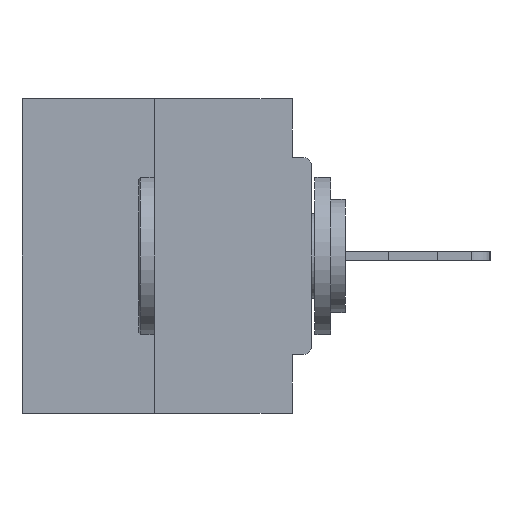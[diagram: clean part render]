
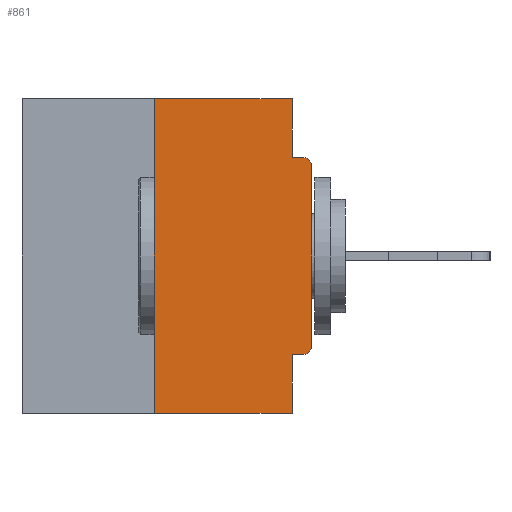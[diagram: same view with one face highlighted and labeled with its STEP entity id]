
A CAD part, left-side view. The second image highlights one B-rep face of the part: STEP entity #861.
In plain terms, the highlighted planar face has unit normal (-1, 0, 0).
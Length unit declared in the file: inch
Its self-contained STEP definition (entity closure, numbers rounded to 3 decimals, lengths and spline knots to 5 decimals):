
#429 = VERTEX_POINT ( 'NONE', #19934 ) ;
#861 = ADVANCED_FACE ( 'NONE', ( #7298 ), #9943, .F. ) ;
#922 = CARTESIAN_POINT ( 'NONE',  ( 0., 0.46, 0. ) ) ;
#953 = LINE ( 'NONE', #10120, #7994 ) ;
#1533 = DIRECTION ( 'NONE',  ( -1., 0., 0. ) ) ;
#2012 = VERTEX_POINT ( 'NONE', #7762 ) ;
#2279 = VERTEX_POINT ( 'NONE', #18960 ) ;
#2913 = DIRECTION ( 'NONE',  ( 0., 0., 1. ) ) ;
#3044 = VERTEX_POINT ( 'NONE', #5951 ) ;
#3590 = LINE ( 'NONE', #22422, #23244 ) ;
#3699 = CARTESIAN_POINT ( 'NONE',  ( 0., 0., -0.1085 ) ) ;
#4119 = EDGE_CURVE ( 'NONE', #4155, #16499, #11860, .T. ) ;
#4155 = VERTEX_POINT ( 'NONE', #9522 ) ;
#4285 = ORIENTED_EDGE ( 'NONE', *, *, #11228, .T. ) ;
#5045 = EDGE_LOOP ( 'NONE', ( #5771, #16058, #4285, #12949, #11270, #27238, #19919, #18585, #28527, #9793 ) ) ;
#5436 = LINE ( 'NONE', #27053, #20895 ) ;
#5771 = ORIENTED_EDGE ( 'NONE', *, *, #6551, .F. ) ;
#5951 = CARTESIAN_POINT ( 'NONE',  ( 0., 0.031, -0.4065 ) ) ;
#6551 = EDGE_CURVE ( 'NONE', #2012, #7113, #3590, .T. ) ;
#6617 = CARTESIAN_POINT ( 'NONE',  ( 0., 0.031, -0.0935 ) ) ;
#6985 = AXIS2_PLACEMENT_3D ( 'NONE', #7805, #1533, #22107 ) ;
#7113 = VERTEX_POINT ( 'NONE', #11018 ) ;
#7218 = VECTOR ( 'NONE', #21047, 39.37008 ) ;
#7298 = FACE_OUTER_BOUND ( 'NONE', #5045, .T. ) ;
#7762 = CARTESIAN_POINT ( 'NONE',  ( 0., 0.25, 0. ) ) ;
#7805 = CARTESIAN_POINT ( 'NONE',  ( 0., 0.015, -0.1085 ) ) ;
#7994 = VECTOR ( 'NONE', #25486, 39.37008 ) ;
#8562 = DIRECTION ( 'NONE',  ( 0., -1., 0. ) ) ;
#9522 = CARTESIAN_POINT ( 'NONE',  ( 0., 0., -0.3915 ) ) ;
#9664 = CARTESIAN_POINT ( 'NONE',  ( 0., 0., 0. ) ) ;
#9793 = ORIENTED_EDGE ( 'NONE', *, *, #26928, .F. ) ;
#9943 = PLANE ( 'NONE',  #16015 ) ;
#10120 = CARTESIAN_POINT ( 'NONE',  ( 0., 0.46, -0.5 ) ) ;
#10135 = LINE ( 'NONE', #22425, #25837 ) ;
#11018 = CARTESIAN_POINT ( 'NONE',  ( 0., 0.031, 0. ) ) ;
#11034 = VECTOR ( 'NONE', #20448, 39.37008 ) ;
#11209 = CARTESIAN_POINT ( 'NONE',  ( 0., 0.015, -0.3915 ) ) ;
#11228 = EDGE_CURVE ( 'NONE', #17692, #16939, #953, .T. ) ;
#11270 = ORIENTED_EDGE ( 'NONE', *, *, #23505, .F. ) ;
#11860 = LINE ( 'NONE', #9664, #7218 ) ;
#12949 = ORIENTED_EDGE ( 'NONE', *, *, #21204, .F. ) ;
#14270 = CARTESIAN_POINT ( 'NONE',  ( 0., 0.25, 0. ) ) ;
#15337 = CARTESIAN_POINT ( 'NONE',  ( 0., 0.031, -0.5 ) ) ;
#16015 = AXIS2_PLACEMENT_3D ( 'NONE', #922, #26295, #19442 ) ;
#16035 = DIRECTION ( 'NONE',  ( 0., 0., -1. ) ) ;
#16058 = ORIENTED_EDGE ( 'NONE', *, *, #16781, .F. ) ;
#16499 = VERTEX_POINT ( 'NONE', #3699 ) ;
#16549 = EDGE_CURVE ( 'NONE', #16499, #429, #27867, .T. ) ;
#16781 = EDGE_CURVE ( 'NONE', #17692, #2012, #23922, .T. ) ;
#16939 = VERTEX_POINT ( 'NONE', #15337 ) ;
#16960 = DIRECTION ( 'NONE',  ( 0., 0., -1. ) ) ;
#17440 = VECTOR ( 'NONE', #2913, 39.37008 ) ;
#17692 = VERTEX_POINT ( 'NONE', #30551 ) ;
#18066 = EDGE_CURVE ( 'NONE', #2279, #4155, #28645, .T. ) ;
#18364 = LINE ( 'NONE', #23180, #30116 ) ;
#18585 = ORIENTED_EDGE ( 'NONE', *, *, #16549, .T. ) ;
#18960 = CARTESIAN_POINT ( 'NONE',  ( 0., 0.015, -0.4065 ) ) ;
#19193 = AXIS2_PLACEMENT_3D ( 'NONE', #11209, #20717, #16035 ) ;
#19442 = DIRECTION ( 'NONE',  ( 0., 0., -1. ) ) ;
#19919 = ORIENTED_EDGE ( 'NONE', *, *, #4119, .T. ) ;
#19934 = CARTESIAN_POINT ( 'NONE',  ( 0., 0.015, -0.0935 ) ) ;
#20448 = DIRECTION ( 'NONE',  ( 0., 1., 0. ) ) ;
#20717 = DIRECTION ( 'NONE',  ( -1., 0., 0. ) ) ;
#20796 = EDGE_CURVE ( 'NONE', #21879, #429, #10135, .T. ) ;
#20895 = VECTOR ( 'NONE', #16960, 39.37008 ) ;
#21047 = DIRECTION ( 'NONE',  ( 0., 0., 1. ) ) ;
#21204 = EDGE_CURVE ( 'NONE', #3044, #16939, #5436, .T. ) ;
#21879 = VERTEX_POINT ( 'NONE', #6617 ) ;
#22107 = DIRECTION ( 'NONE',  ( 0., 0., -1. ) ) ;
#22422 = CARTESIAN_POINT ( 'NONE',  ( 0., 0.46, 0. ) ) ;
#22425 = CARTESIAN_POINT ( 'NONE',  ( 0., 0., -0.0935 ) ) ;
#22612 = LINE ( 'NONE', #29797, #11034 ) ;
#23180 = CARTESIAN_POINT ( 'NONE',  ( 0., 0.031, 0. ) ) ;
#23244 = VECTOR ( 'NONE', #8562, 39.37008 ) ;
#23505 = EDGE_CURVE ( 'NONE', #2279, #3044, #22612, .T. ) ;
#23922 = LINE ( 'NONE', #14270, #17440 ) ;
#25486 = DIRECTION ( 'NONE',  ( 0., -1., 0. ) ) ;
#25837 = VECTOR ( 'NONE', #27259, 39.37008 ) ;
#26295 = DIRECTION ( 'NONE',  ( 1., 0., 0. ) ) ;
#26928 = EDGE_CURVE ( 'NONE', #7113, #21879, #18364, .T. ) ;
#27053 = CARTESIAN_POINT ( 'NONE',  ( 0., 0.031, -0.5 ) ) ;
#27238 = ORIENTED_EDGE ( 'NONE', *, *, #18066, .T. ) ;
#27259 = DIRECTION ( 'NONE',  ( 0., -1., 0. ) ) ;
#27867 = CIRCLE ( 'NONE', #6985, 0.015 ) ;
#28527 = ORIENTED_EDGE ( 'NONE', *, *, #20796, .F. ) ;
#28645 = CIRCLE ( 'NONE', #19193, 0.015 ) ;
#29797 = CARTESIAN_POINT ( 'NONE',  ( 0., 0., -0.4065 ) ) ;
#30116 = VECTOR ( 'NONE', #30353, 39.37008 ) ;
#30353 = DIRECTION ( 'NONE',  ( 0., 0., -1. ) ) ;
#30551 = CARTESIAN_POINT ( 'NONE',  ( 0., 0.25, -0.5 ) ) ;
